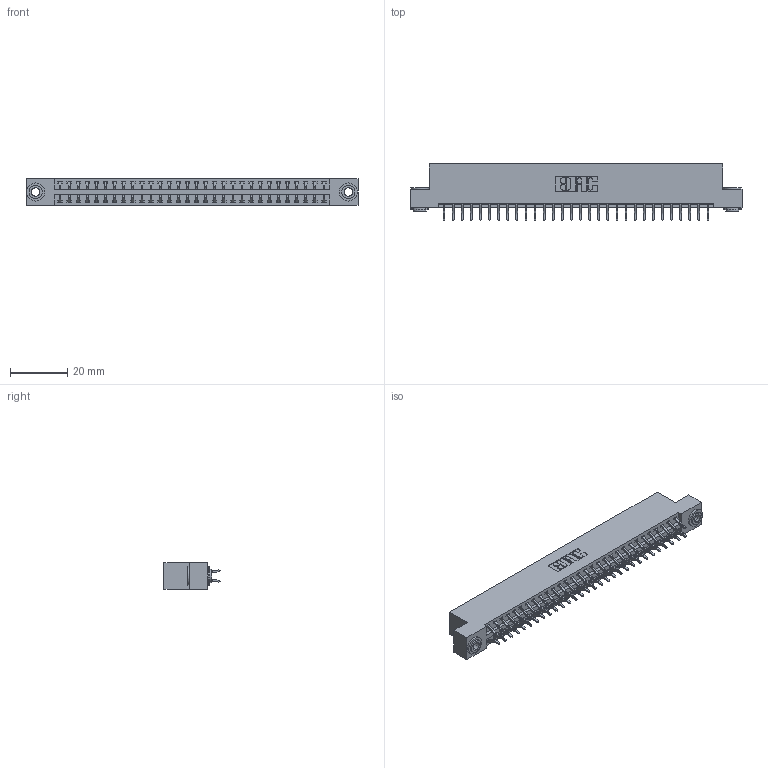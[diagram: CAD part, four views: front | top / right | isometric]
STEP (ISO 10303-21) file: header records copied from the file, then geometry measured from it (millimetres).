
FILE_DESCRIPTION (( 'STEP AP203' ), '1' );
FILE_NAME ('396-060-556-203.STEP', '2019-10-30T16:50:11', ( '' ), ( '' ), 'SwSTEP 2.0', 'SolidWorks 2016', '' );
FILE_SCHEMA (( 'CONFIG_CONTROL_DESIGN' ));
Length unit declared in the file: inch
Products named in the file (4): 345-292-001_556 Tail; 346 Part_Flush Mounting Lugs - 0.156 Dia-TH; 396-060-556-203; 345-250-002_345-250-002-102
Assembly tree (63 placements, depth 2):
  396-060-556-203
    346 Part_Flush Mounting Lugs - 0.156 Dia-TH
    345-292-001_556 Tail  x60
    345-250-002_345-250-002-102  x2
Bounding box: 115.82 x 19.57 x 9.4 mm (x, y, z)
Volume: 11218.1 mm3; surface area: 15389.9 mm2
Topology: 63 solids, 63 shells, 3640 faces, 10785 edges, 7106 vertices
Faces by surface type: plane 2426, cylinder 1206, cone 8
Entity records: 22064 total; most frequent: CARTESIAN_POINT 3643, ORIENTED_EDGE 3558, DIRECTION 3281, EDGE_CURVE 1779, VECTOR 1495, LINE 1495, VERTEX_POINT 1182, AXIS2_PLACEMENT_3D 893
